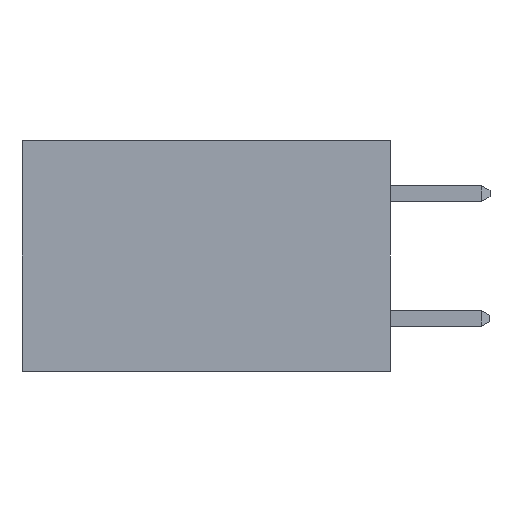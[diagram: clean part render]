
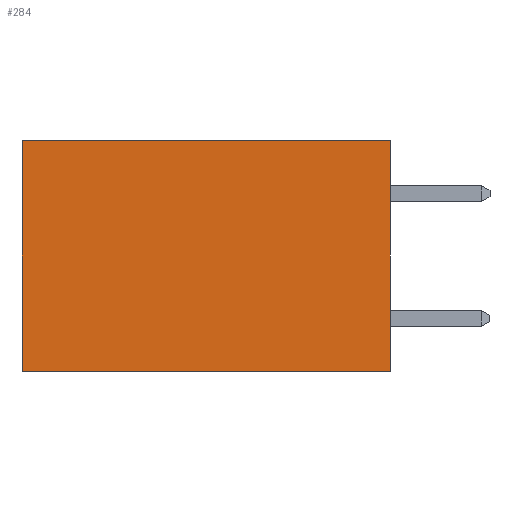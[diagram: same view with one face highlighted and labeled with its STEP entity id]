
A CAD part, left-side view. The second image highlights one B-rep face of the part: STEP entity #284.
In plain terms, the highlighted planar face has unit normal (-1, 0, 0).
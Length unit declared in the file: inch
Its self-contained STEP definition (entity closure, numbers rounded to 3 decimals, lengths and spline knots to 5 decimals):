
#284 = ADVANCED_FACE ( 'NONE', ( #5517 ), #8752, .F. ) ;
#398 = CARTESIAN_POINT ( 'NONE',  ( 0.277, 0., -0.37 ) ) ;
#645 = DIRECTION ( 'NONE',  ( 0., 0., -1. ) ) ;
#1401 = DIRECTION ( 'NONE',  ( 0., 1., 0. ) ) ;
#1730 = CARTESIAN_POINT ( 'NONE',  ( 0.277, 0., -0.37 ) ) ;
#2142 = VERTEX_POINT ( 'NONE', #10565 ) ;
#2906 = EDGE_CURVE ( 'NONE', #10660, #2142, #7787, .T. ) ;
#2981 = LINE ( 'NONE', #10909, #5399 ) ;
#3272 = CARTESIAN_POINT ( 'NONE',  ( 0.277, 0., 0. ) ) ;
#3307 = VECTOR ( 'NONE', #1401, 39.37008 ) ;
#3334 = CARTESIAN_POINT ( 'NONE',  ( 0.277, 0., 0. ) ) ;
#3456 = EDGE_LOOP ( 'NONE', ( #10593, #5637, #5477, #10547 ) ) ;
#3868 = DIRECTION ( 'NONE',  ( 1., 0., 0. ) ) ;
#4228 = LINE ( 'NONE', #6038, #8883 ) ;
#4322 = VERTEX_POINT ( 'NONE', #9289 ) ;
#4432 = DIRECTION ( 'NONE',  ( 0., 0., -1. ) ) ;
#4926 = LINE ( 'NONE', #1730, #11134 ) ;
#5054 = AXIS2_PLACEMENT_3D ( 'NONE', #398, #3868, #4432 ) ;
#5399 = VECTOR ( 'NONE', #10905, 39.37008 ) ;
#5477 = ORIENTED_EDGE ( 'NONE', *, *, #6317, .F. ) ;
#5517 = FACE_OUTER_BOUND ( 'NONE', #3456, .T. ) ;
#5637 = ORIENTED_EDGE ( 'NONE', *, *, #8365, .F. ) ;
#6038 = CARTESIAN_POINT ( 'NONE',  ( 0.277, 0.59, -0.37 ) ) ;
#6317 = EDGE_CURVE ( 'NONE', #10660, #11094, #2981, .T. ) ;
#7787 = LINE ( 'NONE', #3334, #3307 ) ;
#8365 = EDGE_CURVE ( 'NONE', #11094, #4322, #4926, .T. ) ;
#8752 = PLANE ( 'NONE',  #5054 ) ;
#8883 = VECTOR ( 'NONE', #645, 39.37008 ) ;
#9289 = CARTESIAN_POINT ( 'NONE',  ( 0.277, 0.59, -0.37 ) ) ;
#9467 = EDGE_CURVE ( 'NONE', #2142, #4322, #4228, .T. ) ;
#9842 = CARTESIAN_POINT ( 'NONE',  ( 0.277, 0., -0.37 ) ) ;
#10547 = ORIENTED_EDGE ( 'NONE', *, *, #2906, .T. ) ;
#10565 = CARTESIAN_POINT ( 'NONE',  ( 0.277, 0.59, 0. ) ) ;
#10593 = ORIENTED_EDGE ( 'NONE', *, *, #9467, .T. ) ;
#10660 = VERTEX_POINT ( 'NONE', #3272 ) ;
#10905 = DIRECTION ( 'NONE',  ( 0., 0., -1. ) ) ;
#10909 = CARTESIAN_POINT ( 'NONE',  ( 0.277, 0., -0.37 ) ) ;
#11094 = VERTEX_POINT ( 'NONE', #9842 ) ;
#11134 = VECTOR ( 'NONE', #11211, 39.37008 ) ;
#11211 = DIRECTION ( 'NONE',  ( 0., 1., 0. ) ) ;
